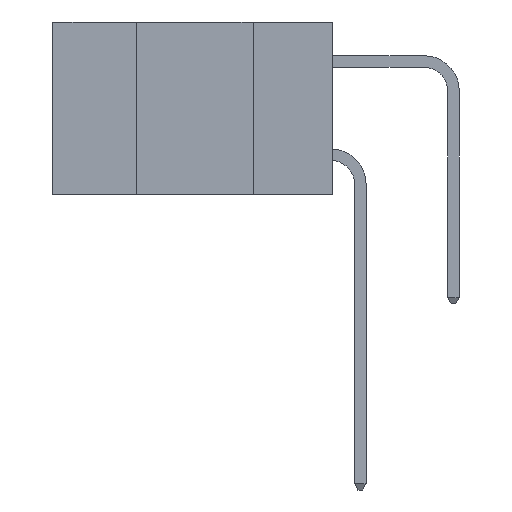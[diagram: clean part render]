
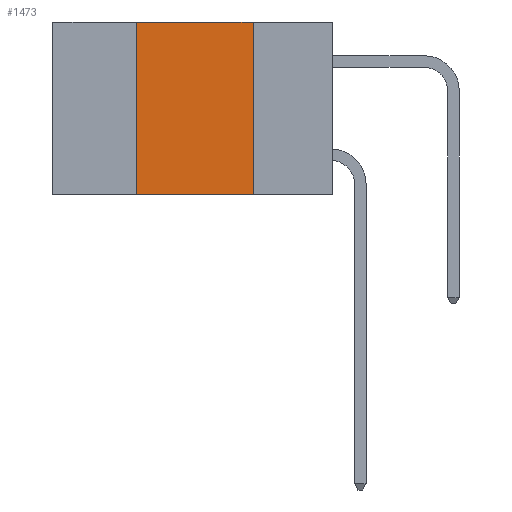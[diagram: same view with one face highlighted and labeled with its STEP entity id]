
A CAD part, left-side view. The second image highlights one B-rep face of the part: STEP entity #1473.
In plain terms, the highlighted planar face has unit normal (-1, 0, 0).
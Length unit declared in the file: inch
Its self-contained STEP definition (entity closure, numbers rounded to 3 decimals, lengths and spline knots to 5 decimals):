
#281 = AXIS2_PLACEMENT_3D ( 'NONE', #6456, #5325, #478 ) ;
#478 = DIRECTION ( 'NONE',  ( 0., 0., -1. ) ) ;
#529 = DIRECTION ( 'NONE',  ( 0., -1., 0. ) ) ;
#1473 = ADVANCED_FACE ( 'NONE', ( #4746 ), #12714, .F. ) ;
#1628 = VECTOR ( 'NONE', #9597, 39.37008 ) ;
#1985 = CARTESIAN_POINT ( 'NONE',  ( 0., 0.17, 0. ) ) ;
#2473 = VERTEX_POINT ( 'NONE', #4410 ) ;
#2606 = CARTESIAN_POINT ( 'NONE',  ( 0., 0.17, -0.37 ) ) ;
#3140 = EDGE_CURVE ( 'NONE', #11465, #5282, #6673, .T. ) ;
#3404 = DIRECTION ( 'NONE',  ( 0., 0., -1. ) ) ;
#3963 = VECTOR ( 'NONE', #529, 39.37008 ) ;
#4345 = LINE ( 'NONE', #9574, #1628 ) ;
#4410 = CARTESIAN_POINT ( 'NONE',  ( 0., 0.42, 0. ) ) ;
#4419 = EDGE_CURVE ( 'NONE', #13093, #2473, #4345, .T. ) ;
#4428 = LINE ( 'NONE', #12529, #6915 ) ;
#4746 = FACE_OUTER_BOUND ( 'NONE', #10335, .T. ) ;
#5168 = ORIENTED_EDGE ( 'NONE', *, *, #12462, .T. ) ;
#5282 = VERTEX_POINT ( 'NONE', #10524 ) ;
#5325 = DIRECTION ( 'NONE',  ( 1., 0., 0. ) ) ;
#5986 = VECTOR ( 'NONE', #3404, 39.37008 ) ;
#6456 = CARTESIAN_POINT ( 'NONE',  ( 0., 0.6, 0. ) ) ;
#6673 = LINE ( 'NONE', #2606, #5986 ) ;
#6769 = CARTESIAN_POINT ( 'NONE',  ( 0., 0.42, -0.37 ) ) ;
#6915 = VECTOR ( 'NONE', #8378, 39.37008 ) ;
#8279 = ORIENTED_EDGE ( 'NONE', *, *, #12207, .F. ) ;
#8378 = DIRECTION ( 'NONE',  ( 0., -1., 0. ) ) ;
#9272 = LINE ( 'NONE', #13046, #3963 ) ;
#9574 = CARTESIAN_POINT ( 'NONE',  ( 0., 0.42, -0.37 ) ) ;
#9597 = DIRECTION ( 'NONE',  ( 0., 0., 1. ) ) ;
#10295 = ORIENTED_EDGE ( 'NONE', *, *, #3140, .F. ) ;
#10335 = EDGE_LOOP ( 'NONE', ( #10295, #8279, #10966, #5168 ) ) ;
#10524 = CARTESIAN_POINT ( 'NONE',  ( 0., 0.17, -0.37 ) ) ;
#10966 = ORIENTED_EDGE ( 'NONE', *, *, #4419, .F. ) ;
#11465 = VERTEX_POINT ( 'NONE', #1985 ) ;
#12207 = EDGE_CURVE ( 'NONE', #2473, #11465, #4428, .T. ) ;
#12462 = EDGE_CURVE ( 'NONE', #13093, #5282, #9272, .T. ) ;
#12529 = CARTESIAN_POINT ( 'NONE',  ( 0., 0.6, 0. ) ) ;
#12714 = PLANE ( 'NONE',  #281 ) ;
#13046 = CARTESIAN_POINT ( 'NONE',  ( 0., 0.6, -0.37 ) ) ;
#13093 = VERTEX_POINT ( 'NONE', #6769 ) ;
